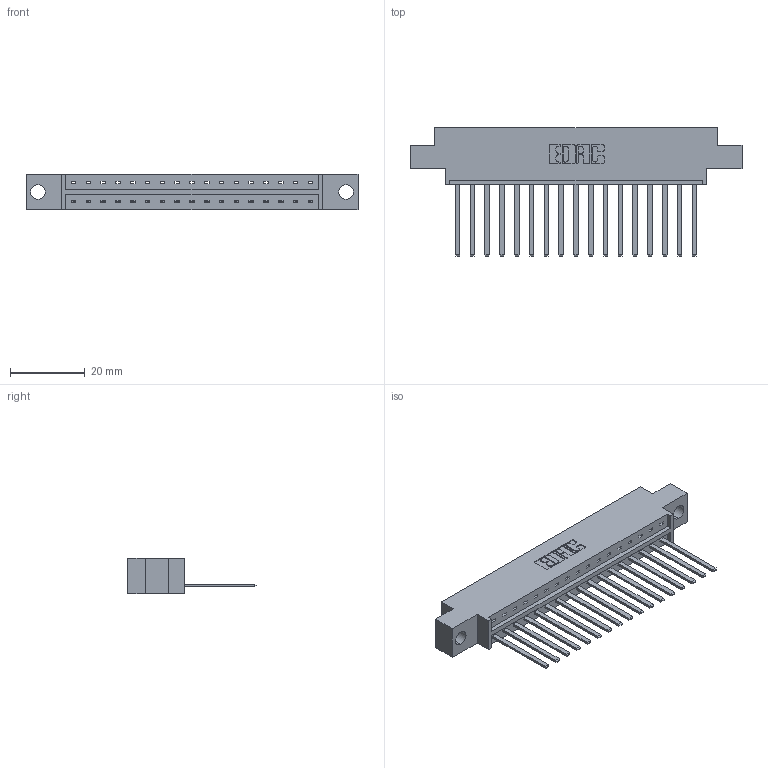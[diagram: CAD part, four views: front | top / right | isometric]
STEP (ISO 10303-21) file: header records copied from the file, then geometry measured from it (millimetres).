
FILE_DESCRIPTION (( 'STEP AP203' ), '1' );
FILE_NAME ('333-017-544-604.STEP', '2019-08-09T12:16:57', ( '' ), ( '' ), 'SwSTEP 2.0', 'SolidWorks 2016', '' );
FILE_SCHEMA (( 'CONFIG_CONTROL_DESIGN' ));
Length unit declared in the file: inch
Products named in the file (3): 333 Part_Offset - .156 Dia - TH; 333-017-544-604; 345-292-001_345-293-144
Assembly tree (18 placements, depth 2):
  333-017-544-604
    333 Part_Offset - .156 Dia - TH
    345-292-001_345-293-144  x17
Bounding box: 88.9 x 34.3 x 9.4 mm (x, y, z)
Volume: 8612.1 mm3; surface area: 9788 mm2
Topology: 18 solids, 18 shells, 1002 faces, 3009 edges, 1982 vertices
Faces by surface type: plane 720, cylinder 282
Entity records: 13577 total; most frequent: CARTESIAN_POINT 2353, ORIENTED_EDGE 2306, DIRECTION 2031, EDGE_CURVE 1153, VECTOR 1029, LINE 1029, VERTEX_POINT 766, AXIS2_PLACEMENT_3D 501
